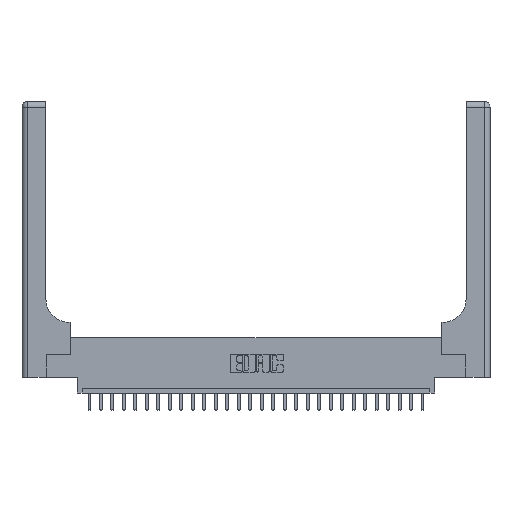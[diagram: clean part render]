
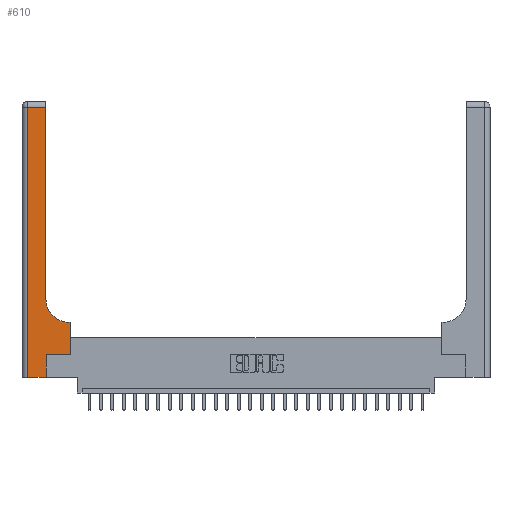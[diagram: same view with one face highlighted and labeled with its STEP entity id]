
A CAD part, top view. The second image highlights one B-rep face of the part: STEP entity #610.
In plain terms, the highlighted planar face has unit normal (0, 0, 1).
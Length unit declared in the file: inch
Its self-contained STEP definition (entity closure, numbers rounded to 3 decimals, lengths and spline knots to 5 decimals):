
#58 = ORIENTED_EDGE ( 'NONE', *, *, #16644, .T. ) ;
#109 = DIRECTION ( 'NONE',  ( 0., 1., 0. ) ) ;
#446 = VECTOR ( 'NONE', #3251, 39.37008 ) ;
#532 = VECTOR ( 'NONE', #7541, 39.37008 ) ;
#610 = ADVANCED_FACE ( 'NONE', ( #7636 ), #1420, .F. ) ;
#1043 = VERTEX_POINT ( 'NONE', #11974 ) ;
#1047 = VERTEX_POINT ( 'NONE', #19721 ) ;
#1099 = DIRECTION ( 'NONE',  ( 0., 0., -1. ) ) ;
#1420 = PLANE ( 'NONE',  #20277 ) ;
#1796 = AXIS2_PLACEMENT_3D ( 'NONE', #21427, #1099, #25546 ) ;
#1855 = VERTEX_POINT ( 'NONE', #18191 ) ;
#2053 = LINE ( 'NONE', #15927, #22645 ) ;
#2741 = ORIENTED_EDGE ( 'NONE', *, *, #16243, .T. ) ;
#3055 = DIRECTION ( 'NONE',  ( 1., 0., 0. ) ) ;
#3251 = DIRECTION ( 'NONE',  ( 0., 1., 0. ) ) ;
#3807 = LINE ( 'NONE', #17931, #15481 ) ;
#4558 = ORIENTED_EDGE ( 'NONE', *, *, #11667, .T. ) ;
#4697 = ORIENTED_EDGE ( 'NONE', *, *, #17110, .T. ) ;
#4746 = VERTEX_POINT ( 'NONE', #23925 ) ;
#4993 = CARTESIAN_POINT ( 'NONE',  ( 0.06, 2.94, 0.37 ) ) ;
#5159 = CARTESIAN_POINT ( 'NONE',  ( 0., 0., 0.37 ) ) ;
#5513 = CARTESIAN_POINT ( 'NONE',  ( 0., 3., 0.37 ) ) ;
#5702 = VECTOR ( 'NONE', #19482, 39.37008 ) ;
#5719 = ORIENTED_EDGE ( 'NONE', *, *, #25111, .T. ) ;
#5846 = ORIENTED_EDGE ( 'NONE', *, *, #15116, .T. ) ;
#6350 = ORIENTED_EDGE ( 'NONE', *, *, #14195, .T. ) ;
#6432 = ORIENTED_EDGE ( 'NONE', *, *, #19199, .T. ) ;
#7322 = VERTEX_POINT ( 'NONE', #26087 ) ;
#7541 = DIRECTION ( 'NONE',  ( 1., 0., 0. ) ) ;
#7636 = FACE_OUTER_BOUND ( 'NONE', #20191, .T. ) ;
#9589 = CARTESIAN_POINT ( 'NONE',  ( 0.265, 0., 0.37 ) ) ;
#10547 = LINE ( 'NONE', #12650, #23296 ) ;
#11469 = DIRECTION ( 'NONE',  ( 0., 0., -1. ) ) ;
#11667 = EDGE_CURVE ( 'NONE', #25969, #1047, #17133, .T. ) ;
#11974 = CARTESIAN_POINT ( 'NONE',  ( 0.265, 0.25, 0.37 ) ) ;
#12650 = CARTESIAN_POINT ( 'NONE',  ( 0.06, 3., 0.37 ) ) ;
#13074 = LINE ( 'NONE', #5159, #18273 ) ;
#13385 = VERTEX_POINT ( 'NONE', #24870 ) ;
#14195 = EDGE_CURVE ( 'NONE', #7322, #25969, #3807, .T. ) ;
#14621 = EDGE_CURVE ( 'NONE', #4746, #21002, #2053, .T. ) ;
#15116 = EDGE_CURVE ( 'NONE', #21443, #1855, #13074, .T. ) ;
#15407 = CARTESIAN_POINT ( 'NONE',  ( 0.26, 3., 0.37 ) ) ;
#15481 = VECTOR ( 'NONE', #109, 39.37008 ) ;
#15927 = CARTESIAN_POINT ( 'NONE',  ( 0., 2.94, 0.37 ) ) ;
#16243 = EDGE_CURVE ( 'NONE', #13385, #4746, #25979, .T. ) ;
#16644 = EDGE_CURVE ( 'NONE', #1047, #13385, #19889, .T. ) ;
#17110 = EDGE_CURVE ( 'NONE', #1043, #7322, #25640, .T. ) ;
#17133 = LINE ( 'NONE', #23327, #5702 ) ;
#17931 = CARTESIAN_POINT ( 'NONE',  ( 0.528, 0.25, 0.37 ) ) ;
#18191 = CARTESIAN_POINT ( 'NONE',  ( 0.265, 0., 0.37 ) ) ;
#18273 = VECTOR ( 'NONE', #3055, 39.37008 ) ;
#19199 = EDGE_CURVE ( 'NONE', #21002, #21443, #10547, .T. ) ;
#19259 = CARTESIAN_POINT ( 'NONE',  ( 0.528, 0.6, 0.37 ) ) ;
#19482 = DIRECTION ( 'NONE',  ( -1., 0., 0. ) ) ;
#19494 = DIRECTION ( 'NONE',  ( -1., 0., 0. ) ) ;
#19721 = CARTESIAN_POINT ( 'NONE',  ( 0.51, 0.6, 0.37 ) ) ;
#19889 = CIRCLE ( 'NONE', #1796, 0.25 ) ;
#20191 = EDGE_LOOP ( 'NONE', ( #2741, #20548, #6432, #5846, #5719, #4697, #6350, #4558, #58 ) ) ;
#20277 = AXIS2_PLACEMENT_3D ( 'NONE', #5513, #11469, #19494 ) ;
#20548 = ORIENTED_EDGE ( 'NONE', *, *, #14621, .T. ) ;
#21002 = VERTEX_POINT ( 'NONE', #4993 ) ;
#21427 = CARTESIAN_POINT ( 'NONE',  ( 0.51, 0.85, 0.37 ) ) ;
#21443 = VERTEX_POINT ( 'NONE', #24659 ) ;
#21456 = DIRECTION ( 'NONE',  ( 0., 1., 0. ) ) ;
#21984 = VECTOR ( 'NONE', #21456, 39.37008 ) ;
#22545 = DIRECTION ( 'NONE',  ( 0., -1., 0. ) ) ;
#22645 = VECTOR ( 'NONE', #26095, 39.37008 ) ;
#23296 = VECTOR ( 'NONE', #22545, 39.37008 ) ;
#23327 = CARTESIAN_POINT ( 'NONE',  ( 0.26, 0.6, 0.37 ) ) ;
#23378 = CARTESIAN_POINT ( 'NONE',  ( 0.265, 0.25, 0.37 ) ) ;
#23925 = CARTESIAN_POINT ( 'NONE',  ( 0.26, 2.94, 0.37 ) ) ;
#24659 = CARTESIAN_POINT ( 'NONE',  ( 0.06, 0., 0.37 ) ) ;
#24870 = CARTESIAN_POINT ( 'NONE',  ( 0.26, 0.85, 0.37 ) ) ;
#25111 = EDGE_CURVE ( 'NONE', #1855, #1043, #25297, .T. ) ;
#25297 = LINE ( 'NONE', #9589, #446 ) ;
#25546 = DIRECTION ( 'NONE',  ( 1., 0., 0. ) ) ;
#25640 = LINE ( 'NONE', #23378, #532 ) ;
#25969 = VERTEX_POINT ( 'NONE', #19259 ) ;
#25979 = LINE ( 'NONE', #15407, #21984 ) ;
#26087 = CARTESIAN_POINT ( 'NONE',  ( 0.528, 0.25, 0.37 ) ) ;
#26095 = DIRECTION ( 'NONE',  ( -1., 0., 0. ) ) ;
